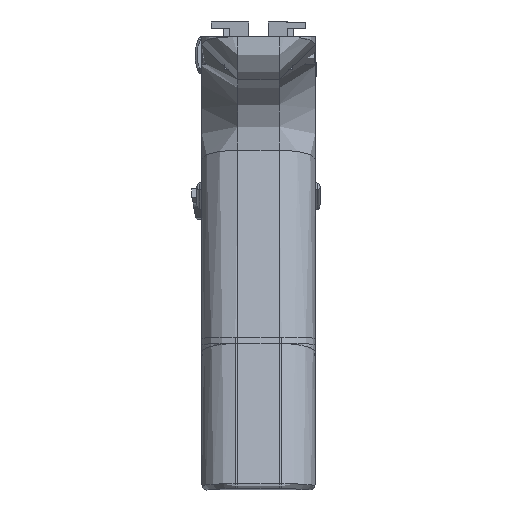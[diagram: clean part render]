
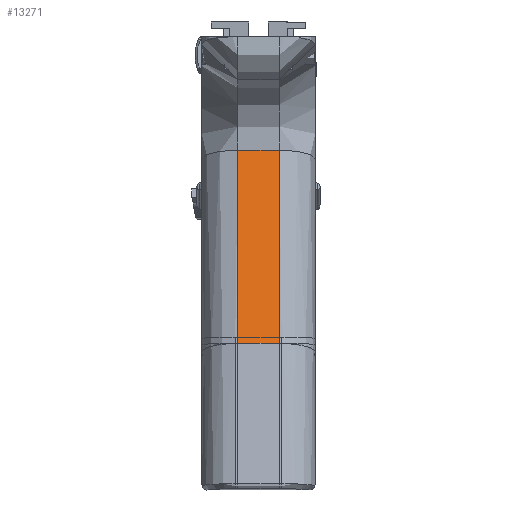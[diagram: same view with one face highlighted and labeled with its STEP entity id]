
A CAD part, front view. The second image highlights one B-rep face of the part: STEP entity #13271.
In plain terms, the highlighted face is planar.
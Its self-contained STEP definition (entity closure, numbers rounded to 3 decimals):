
#1046=PLANE('',#14477);
#1665=FACE_OUTER_BOUND('',#2434,.T.);
#2434=EDGE_LOOP('',(#11532,#11533,#11534,#11535));
#3451=LINE('',#23793,#4624);
#3598=LINE('',#24536,#4771);
#3599=LINE('',#24539,#4772);
#3600=LINE('',#24540,#4773);
#4624=VECTOR('',#17135,10.);
#4771=VECTOR('',#17526,10.);
#4772=VECTOR('',#17529,10.);
#4773=VECTOR('',#17530,10.);
#6239=VERTEX_POINT('',#23789);
#6240=VERTEX_POINT('',#23791);
#6367=VERTEX_POINT('',#24514);
#6370=VERTEX_POINT('',#24538);
#7954=EDGE_CURVE('',#6239,#6240,#3451,.T.);
#8168=EDGE_CURVE('',#6239,#6367,#3598,.T.);
#8169=EDGE_CURVE('',#6370,#6240,#3599,.T.);
#8170=EDGE_CURVE('',#6367,#6370,#3600,.T.);
#11532=ORIENTED_EDGE('',*,*,#8169,.F.);
#11533=ORIENTED_EDGE('',*,*,#8170,.F.);
#11534=ORIENTED_EDGE('',*,*,#8168,.F.);
#11535=ORIENTED_EDGE('',*,*,#7954,.T.);
#13271=ADVANCED_FACE('',(#1665),#1046,.T.);
#14477=AXIS2_PLACEMENT_3D('',#24537,#17527,#17528);
#17135=DIRECTION('',(0.,-0.249,0.969));
#17526=DIRECTION('',(-1.,0.,0.));
#17527=DIRECTION('center_axis',(0.,-0.969,
-0.249));
#17528=DIRECTION('ref_axis',(0.,-0.249,0.969));
#17529=DIRECTION('',(1.,0.,0.));
#17530=DIRECTION('',(0.,-0.249,0.969));
#23789=CARTESIAN_POINT('',(13.45,-71.634,19.877));
#23791=CARTESIAN_POINT('',(13.45,-83.628,66.536));
#23793=CARTESIAN_POINT('',(13.45,-83.554,66.245));
#24514=CARTESIAN_POINT('',(3.45,-71.634,19.877));
#24536=CARTESIAN_POINT('',(22.175,-71.634,19.877));
#24537=CARTESIAN_POINT('Origin',(22.175,-71.634,19.877));
#24538=CARTESIAN_POINT('',(3.45,-83.628,66.536));
#24539=CARTESIAN_POINT('',(22.175,-83.628,66.536));
#24540=CARTESIAN_POINT('',(3.45,-83.554,66.245));
